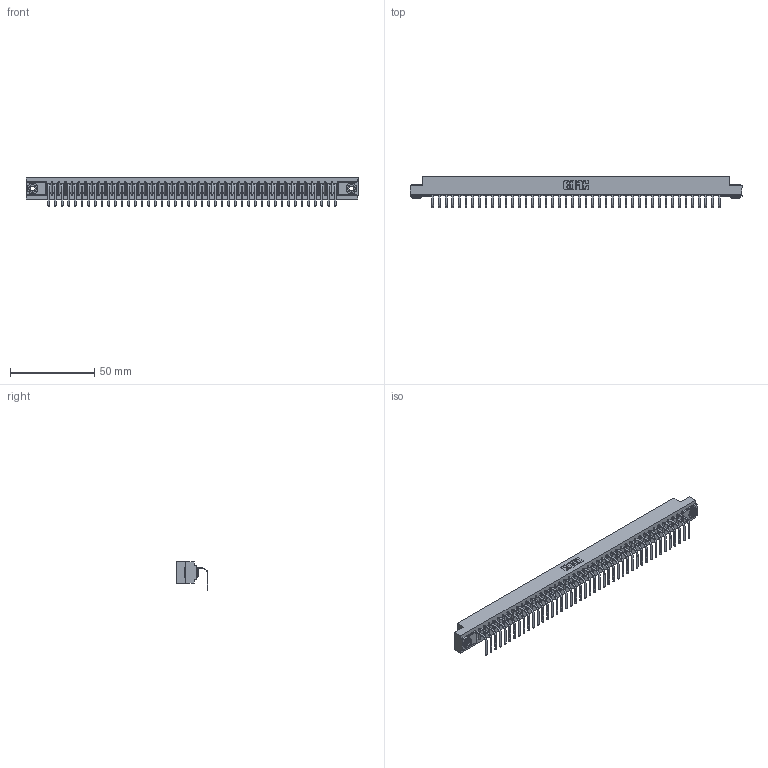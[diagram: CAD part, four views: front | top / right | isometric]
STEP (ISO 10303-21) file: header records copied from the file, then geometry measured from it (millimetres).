
FILE_DESCRIPTION (( 'STEP AP203' ), '1' );
FILE_NAME ('357-044-558-103.STEP', '2022-07-13T17:54:08', ( '' ), ( '' ), 'SwSTEP 2.0', 'SolidWorks 2020', '' );
FILE_SCHEMA (( 'CONFIG_CONTROL_DESIGN' ));
Length unit declared in the file: inch
Products named in the file (4): 307 Part_.156 Dia Mounting Holes; 345-250-002_345-250-002-102; 357-044-558-103; 307-290-001_558 - 2 (Single)
Assembly tree (47 placements, depth 2):
  357-044-558-103
    307 Part_.156 Dia Mounting Holes
    307-290-001_558 - 2 (Single)  x44
    345-250-002_345-250-002-102  x2
Bounding box: 197.36 x 18.78 x 16.8 mm (x, y, z)
Volume: 20682.1 mm3; surface area: 23349.3 mm2
Topology: 47 solids, 47 shells, 2855 faces, 8091 edges, 5210 vertices
Faces by surface type: plane 1810, cylinder 947, sphere 90, cone 8
Entity records: 38643 total; most frequent: CARTESIAN_POINT 6489, ORIENTED_EDGE 6466, DIRECTION 6325, EDGE_CURVE 3233, LINE 2473, VECTOR 2473, VERTEX_POINT 2090, AXIS2_PLACEMENT_3D 1926
